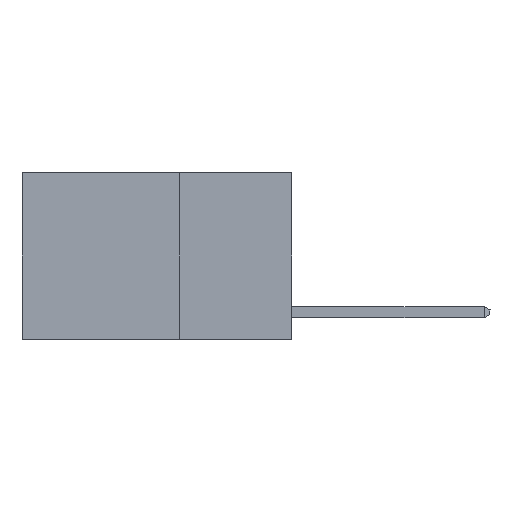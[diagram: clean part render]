
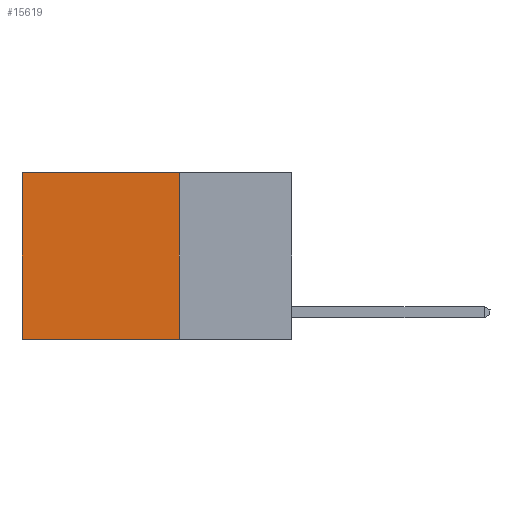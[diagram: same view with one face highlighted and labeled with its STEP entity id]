
A CAD part, left-side view. The second image highlights one B-rep face of the part: STEP entity #15619.
In plain terms, the highlighted planar face has unit normal (-1, 0, 0).
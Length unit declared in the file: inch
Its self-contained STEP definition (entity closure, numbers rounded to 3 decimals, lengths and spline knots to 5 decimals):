
#552 = CARTESIAN_POINT ( 'NONE',  ( 0.2625, 0.25, -0.37 ) ) ;
#611 = EDGE_CURVE ( 'NONE', #6456, #14323, #15211, .T. ) ;
#821 = CARTESIAN_POINT ( 'NONE',  ( 0.2625, 0.6, 0. ) ) ;
#1434 = VERTEX_POINT ( 'NONE', #14450 ) ;
#1520 = VERTEX_POINT ( 'NONE', #7799 ) ;
#1624 = DIRECTION ( 'NONE',  ( 0., 0., -1. ) ) ;
#1996 = DIRECTION ( 'NONE',  ( 0., 0., -1. ) ) ;
#2063 = LINE ( 'NONE', #16275, #5913 ) ;
#2701 = EDGE_CURVE ( 'NONE', #1520, #1434, #6665, .T. ) ;
#4120 = ORIENTED_EDGE ( 'NONE', *, *, #611, .T. ) ;
#4719 = LINE ( 'NONE', #552, #7137 ) ;
#5913 = VECTOR ( 'NONE', #11741, 39.37008 ) ;
#6456 = VERTEX_POINT ( 'NONE', #12071 ) ;
#6665 = LINE ( 'NONE', #18018, #8176 ) ;
#7137 = VECTOR ( 'NONE', #14855, 39.37008 ) ;
#7245 = ORIENTED_EDGE ( 'NONE', *, *, #18057, .T. ) ;
#7799 = CARTESIAN_POINT ( 'NONE',  ( 0.2625, 0.25, 0. ) ) ;
#8176 = VECTOR ( 'NONE', #1996, 39.37008 ) ;
#8493 = CARTESIAN_POINT ( 'NONE',  ( 0.2625, 0.6, -0.37 ) ) ;
#9895 = PLANE ( 'NONE',  #13438 ) ;
#10266 = CARTESIAN_POINT ( 'NONE',  ( 0.2625, 0.25, 0. ) ) ;
#11741 = DIRECTION ( 'NONE',  ( 0., 1., 0. ) ) ;
#12071 = CARTESIAN_POINT ( 'NONE',  ( 0.2625, 0.6, 0. ) ) ;
#13127 = FACE_OUTER_BOUND ( 'NONE', #15450, .T. ) ;
#13438 = AXIS2_PLACEMENT_3D ( 'NONE', #10266, #14629, #1624 ) ;
#13686 = ORIENTED_EDGE ( 'NONE', *, *, #17923, .F. ) ;
#14323 = VERTEX_POINT ( 'NONE', #8493 ) ;
#14450 = CARTESIAN_POINT ( 'NONE',  ( 0.2625, 0.25, -0.37 ) ) ;
#14629 = DIRECTION ( 'NONE',  ( 1., 0., 0. ) ) ;
#14855 = DIRECTION ( 'NONE',  ( 0., 1., 0. ) ) ;
#15029 = DIRECTION ( 'NONE',  ( 0., 0., -1. ) ) ;
#15211 = LINE ( 'NONE', #821, #16554 ) ;
#15450 = EDGE_LOOP ( 'NONE', ( #4120, #13686, #18032, #7245 ) ) ;
#15619 = ADVANCED_FACE ( 'NONE', ( #13127 ), #9895, .F. ) ;
#16275 = CARTESIAN_POINT ( 'NONE',  ( 0.2625, 0.25, 0. ) ) ;
#16554 = VECTOR ( 'NONE', #15029, 39.37008 ) ;
#17923 = EDGE_CURVE ( 'NONE', #1434, #14323, #4719, .T. ) ;
#18018 = CARTESIAN_POINT ( 'NONE',  ( 0.2625, 0.25, 0. ) ) ;
#18032 = ORIENTED_EDGE ( 'NONE', *, *, #2701, .F. ) ;
#18057 = EDGE_CURVE ( 'NONE', #1520, #6456, #2063, .T. ) ;
